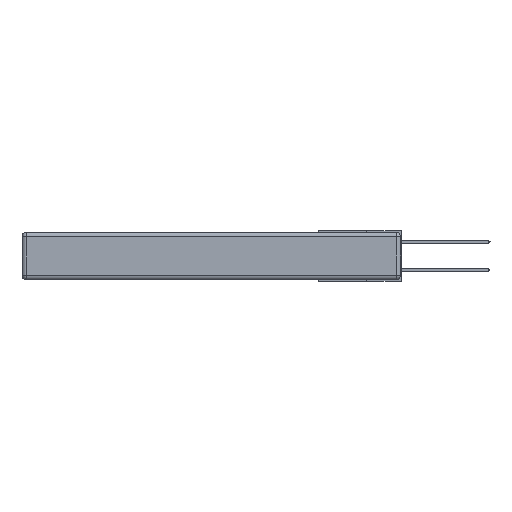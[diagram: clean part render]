
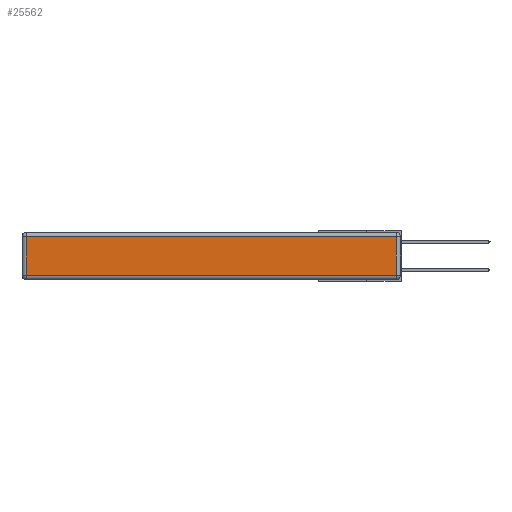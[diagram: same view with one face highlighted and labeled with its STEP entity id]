
A CAD part, left-side view. The second image highlights one B-rep face of the part: STEP entity #25562.
In plain terms, the highlighted planar face has unit normal (-1, 0, 0).
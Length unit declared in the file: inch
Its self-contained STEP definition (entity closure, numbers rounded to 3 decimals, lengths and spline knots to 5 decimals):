
#862 = CARTESIAN_POINT ( 'NONE',  ( 0., 2.75, -0.03 ) ) ;
#1015 = DIRECTION ( 'NONE',  ( 0., 0., 1. ) ) ;
#1477 = ORIENTED_EDGE ( 'NONE', *, *, #18955, .T. ) ;
#2562 = ORIENTED_EDGE ( 'NONE', *, *, #12873, .T. ) ;
#2618 = LINE ( 'NONE', #10016, #22468 ) ;
#3008 = VERTEX_POINT ( 'NONE', #22555 ) ;
#3907 = AXIS2_PLACEMENT_3D ( 'NONE', #11299, #7143, #20192 ) ;
#5236 = CARTESIAN_POINT ( 'NONE',  ( 0., 0., -0.313 ) ) ;
#6964 = PLANE ( 'NONE',  #3907 ) ;
#6992 = DIRECTION ( 'NONE',  ( 0., 1., 0. ) ) ;
#7143 = DIRECTION ( 'NONE',  ( -1., 0., 0. ) ) ;
#7726 = FACE_OUTER_BOUND ( 'NONE', #17229, .T. ) ;
#10016 = CARTESIAN_POINT ( 'NONE',  ( 0., 2.72, -0.343 ) ) ;
#10265 = VERTEX_POINT ( 'NONE', #18858 ) ;
#11247 = ORIENTED_EDGE ( 'NONE', *, *, #21418, .T. ) ;
#11299 = CARTESIAN_POINT ( 'NONE',  ( 0., 0., -0.343 ) ) ;
#11941 = CARTESIAN_POINT ( 'NONE',  ( 0., 0.03, -0.343 ) ) ;
#12873 = EDGE_CURVE ( 'NONE', #15425, #24723, #17855, .T. ) ;
#13938 = LINE ( 'NONE', #862, #14304 ) ;
#14304 = VECTOR ( 'NONE', #6992, 39.37008 ) ;
#15425 = VERTEX_POINT ( 'NONE', #15596 ) ;
#15596 = CARTESIAN_POINT ( 'NONE',  ( 0., 2.72, -0.313 ) ) ;
#17229 = EDGE_LOOP ( 'NONE', ( #2562, #26052, #1477, #11247 ) ) ;
#17855 = LINE ( 'NONE', #5236, #27652 ) ;
#18858 = CARTESIAN_POINT ( 'NONE',  ( 0., 2.72, -0.03 ) ) ;
#18955 = EDGE_CURVE ( 'NONE', #3008, #10265, #13938, .T. ) ;
#19634 = LINE ( 'NONE', #11941, #24687 ) ;
#20192 = DIRECTION ( 'NONE',  ( 0., 0., 1. ) ) ;
#21418 = EDGE_CURVE ( 'NONE', #10265, #15425, #2618, .T. ) ;
#22385 = DIRECTION ( 'NONE',  ( 0., -1., 0. ) ) ;
#22468 = VECTOR ( 'NONE', #23292, 39.37008 ) ;
#22555 = CARTESIAN_POINT ( 'NONE',  ( 0., 0.03, -0.03 ) ) ;
#22626 = CARTESIAN_POINT ( 'NONE',  ( 0., 0.03, -0.313 ) ) ;
#23292 = DIRECTION ( 'NONE',  ( 0., 0., -1. ) ) ;
#23851 = EDGE_CURVE ( 'NONE', #24723, #3008, #19634, .T. ) ;
#24687 = VECTOR ( 'NONE', #1015, 39.37008 ) ;
#24723 = VERTEX_POINT ( 'NONE', #22626 ) ;
#25562 = ADVANCED_FACE ( 'NONE', ( #7726 ), #6964, .T. ) ;
#26052 = ORIENTED_EDGE ( 'NONE', *, *, #23851, .T. ) ;
#27652 = VECTOR ( 'NONE', #22385, 39.37008 ) ;
